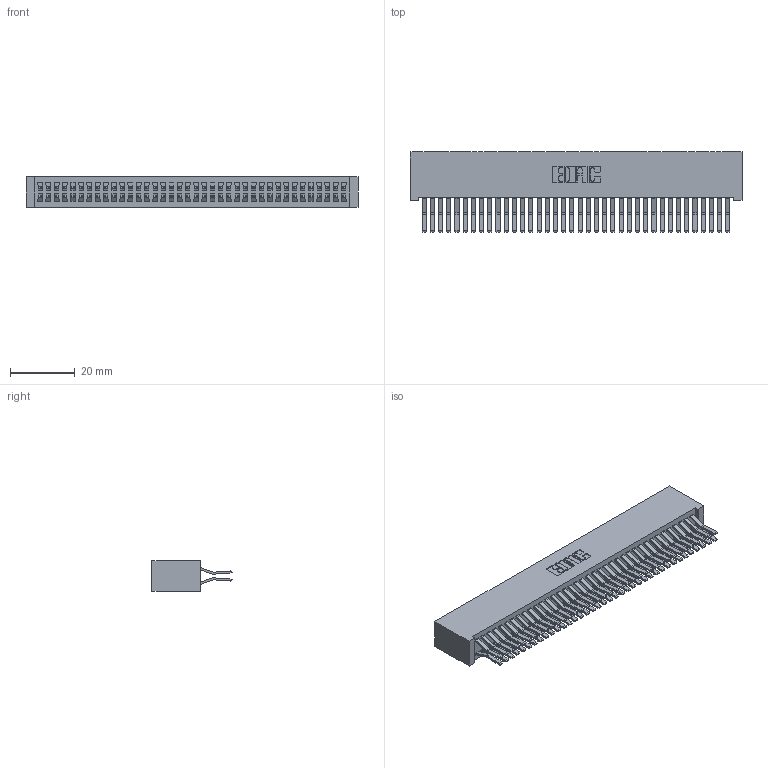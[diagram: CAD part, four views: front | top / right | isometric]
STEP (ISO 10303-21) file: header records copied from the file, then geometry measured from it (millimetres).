
FILE_DESCRIPTION (( 'STEP AP203' ), '1' );
FILE_NAME ('342-076-560-201.STEP', '2019-10-04T10:57:23', ( '' ), ( '' ), 'SwSTEP 2.0', 'SolidWorks 2016', '' );
FILE_SCHEMA (( 'CONFIG_CONTROL_DESIGN' ));
Length unit declared in the file: inch
Products named in the file (3): 342 Part_Lugless; 345-292-001_560 Tail; 342-076-560-201
Assembly tree (77 placements, depth 2):
  342-076-560-201
    342 Part_Lugless
    345-292-001_560 Tail  x76
Bounding box: 102.77 x 24.78 x 9.4 mm (x, y, z)
Volume: 10153.3 mm3; surface area: 18071.1 mm2
Topology: 77 solids, 77 shells, 4206 faces, 12511 edges, 8238 vertices
Faces by surface type: plane 2798, cylinder 1408
Entity records: 24643 total; most frequent: CARTESIAN_POINT 4086, ORIENTED_EDGE 4022, DIRECTION 3495, EDGE_CURVE 2011, LINE 1887, VECTOR 1887, VERTEX_POINT 1338, AXIS2_PLACEMENT_3D 804
